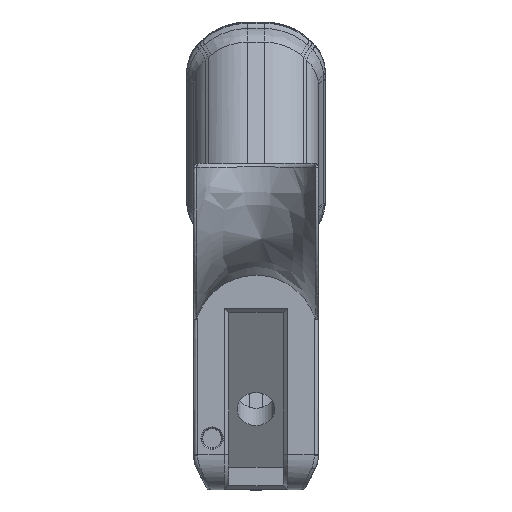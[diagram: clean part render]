
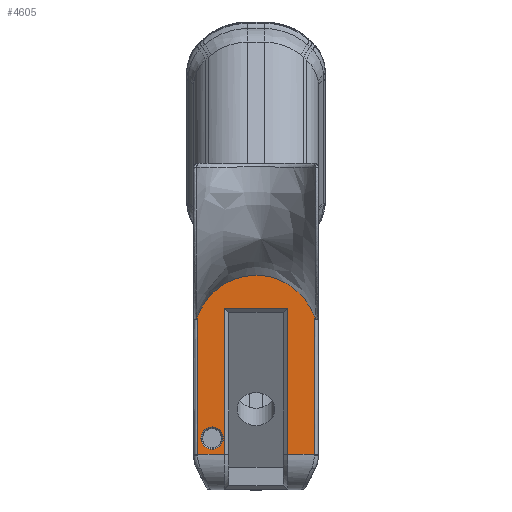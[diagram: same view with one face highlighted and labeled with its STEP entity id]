
A CAD part, top view. The second image highlights one B-rep face of the part: STEP entity #4605.
In plain terms, the highlighted planar face has unit normal (0, 0, 1).
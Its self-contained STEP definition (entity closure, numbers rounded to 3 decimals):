
#37=FACE_BOUND('',#1317,.T.);
#280=B_SPLINE_CURVE_WITH_KNOTS('',3,(#9452,#9453,#9454,#9455,#9456,#9457,
#9458,#9459,#9460,#9461,#9462,#9463),.UNSPECIFIED.,.F.,.F.,(4,2,2,2,2,4),
(1.71,1.762,2.19,2.624,3.022,
3.106),.UNSPECIFIED.);
#281=B_SPLINE_CURVE_WITH_KNOTS('',3,(#9465,#9466,#9467,#9468,#9469,#9470,
#9471,#9472,#9473,#9474),.UNSPECIFIED.,.F.,.F.,(4,2,2,2,4),(0.313,
0.444,0.89,1.331,1.71),
 .UNSPECIFIED.);
#341=B_SPLINE_CURVE_WITH_KNOTS('',3,(#11192,#11193,#11194,#11195),
 .UNSPECIFIED.,.F.,.F.,(4,4),(-2.445,-0.005),
 .UNSPECIFIED.);
#343=B_SPLINE_CURVE_WITH_KNOTS('',3,(#11303,#11304,#11305,#11306),
 .UNSPECIFIED.,.F.,.F.,(4,4),(-7.406,-4.966),
 .UNSPECIFIED.);
#582=CIRCLE('',#4965,2.);
#1005=FACE_OUTER_BOUND('',#1316,.T.);
#1316=EDGE_LOOP('',(#3870,#3871,#3872,#3873,#3874,#3875,#3876,#3877,#3878));
#1317=EDGE_LOOP('',(#3879));
#1539=LINE('',#9327,#1734);
#1545=LINE('',#9338,#1740);
#1550=LINE('',#9356,#1745);
#1559=LINE('',#11300,#1754);
#1560=LINE('',#11302,#1755);
#1734=VECTOR('',#5638,10.);
#1740=VECTOR('',#5648,10.);
#1745=VECTOR('',#5661,10.);
#1754=VECTOR('',#5726,10.);
#1755=VECTOR('',#5727,10.);
#2053=VERTEX_POINT('',#9325);
#2054=VERTEX_POINT('',#9326);
#2057=VERTEX_POINT('',#9337);
#2061=VERTEX_POINT('',#9355);
#2068=VERTEX_POINT('',#9446);
#2069=VERTEX_POINT('',#9451);
#2070=VERTEX_POINT('',#9464);
#2124=VERTEX_POINT('',#11299);
#2125=VERTEX_POINT('',#11301);
#2126=VERTEX_POINT('',#11307);
#2632=EDGE_CURVE('',#2053,#2054,#1539,.T.);
#2638=EDGE_CURVE('',#2057,#2053,#1545,.T.);
#2645=EDGE_CURVE('',#2061,#2054,#1550,.T.);
#2653=EDGE_CURVE('',#2069,#2068,#280,.T.);
#2654=EDGE_CURVE('',#2070,#2069,#281,.T.);
#2740=EDGE_CURVE('',#2061,#2068,#341,.T.);
#2742=EDGE_CURVE('',#2124,#2057,#1559,.T.);
#2743=EDGE_CURVE('',#2125,#2124,#1560,.T.);
#2744=EDGE_CURVE('',#2070,#2125,#343,.T.);
#2745=EDGE_CURVE('',#2126,#2126,#582,.T.);
#3870=ORIENTED_EDGE('',*,*,#2653,.T.);
#3871=ORIENTED_EDGE('',*,*,#2740,.F.);
#3872=ORIENTED_EDGE('',*,*,#2645,.T.);
#3873=ORIENTED_EDGE('',*,*,#2632,.F.);
#3874=ORIENTED_EDGE('',*,*,#2638,.F.);
#3875=ORIENTED_EDGE('',*,*,#2742,.F.);
#3876=ORIENTED_EDGE('',*,*,#2743,.F.);
#3877=ORIENTED_EDGE('',*,*,#2744,.F.);
#3878=ORIENTED_EDGE('',*,*,#2654,.T.);
#3879=ORIENTED_EDGE('',*,*,#2745,.F.);
#4368=PLANE('',#4964);
#4605=ADVANCED_FACE('',(#1005,#37),#4368,.T.);
#4964=AXIS2_PLACEMENT_3D('',#11298,#5724,#5725);
#4965=AXIS2_PLACEMENT_3D('',#11308,#5728,#5729);
#5638=DIRECTION('',(0.,-1.,0.));
#5648=DIRECTION('',(-1.,0.,0.));
#5661=DIRECTION('',(1.,0.,0.));
#5724=DIRECTION('center_axis',(0.,0.,
1.));
#5725=DIRECTION('ref_axis',(0.,-1.,0.));
#5726=DIRECTION('',(0.,1.,0.));
#5727=DIRECTION('',(-1.,0.,0.));
#5728=DIRECTION('center_axis',(0.,0.,
1.));
#5729=DIRECTION('ref_axis',(1.,0.,0.));
#9325=CARTESIAN_POINT('',(18.417,-117.318,28.406));
#9326=CARTESIAN_POINT('',(18.417,-143.468,28.406));
#9327=CARTESIAN_POINT('',(18.417,-114.618,28.406));
#9337=CARTESIAN_POINT('',(29.746,-117.318,28.406));
#9338=CARTESIAN_POINT('',(24.173,-117.318,28.406));
#9355=CARTESIAN_POINT('',(13.65,-143.468,28.406));
#9356=CARTESIAN_POINT('',(28.956,-143.468,28.406));
#9446=CARTESIAN_POINT('',(13.518,-119.073,28.406));
#9451=CARTESIAN_POINT('',(24.081,-111.416,28.406));
#9452=CARTESIAN_POINT('Ctrl Pts',(24.081,-111.416,28.406));
#9453=CARTESIAN_POINT('Ctrl Pts',(23.907,-111.416,28.406));
#9454=CARTESIAN_POINT('Ctrl Pts',(23.733,-111.42,28.406));
#9455=CARTESIAN_POINT('Ctrl Pts',(22.136,-111.497,28.406));
#9456=CARTESIAN_POINT('Ctrl Pts',(20.743,-111.842,28.406));
#9457=CARTESIAN_POINT('Ctrl Pts',(18.138,-113.053,28.406));
#9458=CARTESIAN_POINT('Ctrl Pts',(16.956,-113.915,28.406));
#9459=CARTESIAN_POINT('Ctrl Pts',(15.066,-115.943,28.406));
#9460=CARTESIAN_POINT('Ctrl Pts',(14.34,-117.063,28.406));
#9461=CARTESIAN_POINT('Ctrl Pts',(13.71,-118.541,28.406));
#9462=CARTESIAN_POINT('Ctrl Pts',(13.609,-118.805,28.406));
#9463=CARTESIAN_POINT('Ctrl Pts',(13.518,-119.073,28.406));
#9464=CARTESIAN_POINT('',(34.645,-119.073,28.406));
#9465=CARTESIAN_POINT('Ctrl Pts',(34.645,-119.073,28.406));
#9466=CARTESIAN_POINT('Ctrl Pts',(34.504,-118.659,28.406));
#9467=CARTESIAN_POINT('Ctrl Pts',(34.339,-118.252,28.406));
#9468=CARTESIAN_POINT('Ctrl Pts',(33.514,-116.514,28.406));
#9469=CARTESIAN_POINT('Ctrl Pts',(32.621,-115.308,28.406));
#9470=CARTESIAN_POINT('Ctrl Pts',(30.434,-113.323,28.406));
#9471=CARTESIAN_POINT('Ctrl Pts',(29.164,-112.556,28.406));
#9472=CARTESIAN_POINT('Ctrl Pts',(26.592,-111.634,28.406));
#9473=CARTESIAN_POINT('Ctrl Pts',(25.341,-111.416,28.406));
#9474=CARTESIAN_POINT('Ctrl Pts',(24.081,-111.416,28.406));
#11192=CARTESIAN_POINT('Ctrl Pts',(13.65,-143.468,28.406));
#11193=CARTESIAN_POINT('Ctrl Pts',(13.606,-135.336,28.406));
#11194=CARTESIAN_POINT('Ctrl Pts',(13.562,-127.206,28.406));
#11195=CARTESIAN_POINT('Ctrl Pts',(13.518,-119.073,28.406));
#11298=CARTESIAN_POINT('Origin',(19.207,-112.624,28.406));
#11299=CARTESIAN_POINT('',(29.746,-143.468,28.406));
#11300=CARTESIAN_POINT('',(29.746,-114.618,28.406));
#11301=CARTESIAN_POINT('',(34.513,-143.468,28.406));
#11302=CARTESIAN_POINT('',(19.207,-143.468,28.406));
#11303=CARTESIAN_POINT('Ctrl Pts',(34.645,-119.073,28.406));
#11304=CARTESIAN_POINT('Ctrl Pts',(34.601,-127.206,28.406));
#11305=CARTESIAN_POINT('Ctrl Pts',(34.557,-135.336,28.406));
#11306=CARTESIAN_POINT('Ctrl Pts',(34.513,-143.468,28.406));
#11307=CARTESIAN_POINT('',(14.205,-140.572,28.406));
#11308=CARTESIAN_POINT('Origin',(16.205,-140.572,28.406));
